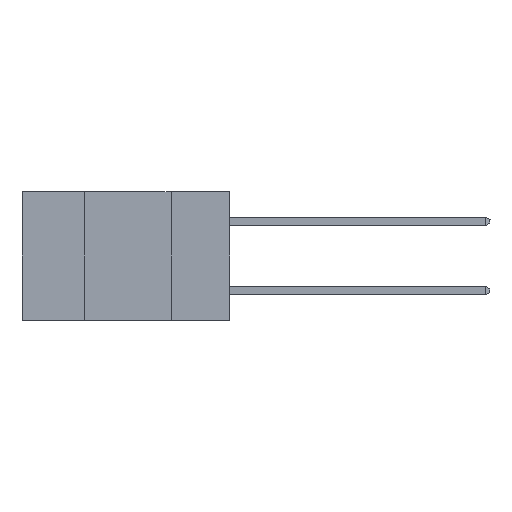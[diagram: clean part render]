
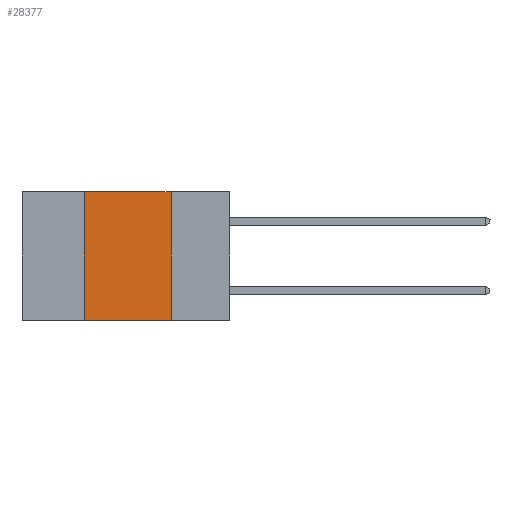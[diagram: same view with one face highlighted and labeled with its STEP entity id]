
A CAD part, left-side view. The second image highlights one B-rep face of the part: STEP entity #28377.
In plain terms, the highlighted planar face has unit normal (-1, 0, 0).
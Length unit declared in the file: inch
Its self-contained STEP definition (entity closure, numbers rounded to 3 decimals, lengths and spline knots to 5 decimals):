
#47 = PLANE ( 'NONE',  #2094 ) ;
#1327 = LINE ( 'NONE', #29027, #18824 ) ;
#1654 = CARTESIAN_POINT ( 'NONE',  ( 0., 0.17, -0.37 ) ) ;
#2094 = AXIS2_PLACEMENT_3D ( 'NONE', #13834, #7036, #9149 ) ;
#2950 = FACE_OUTER_BOUND ( 'NONE', #19973, .T. ) ;
#3147 = VERTEX_POINT ( 'NONE', #9108 ) ;
#4509 = ORIENTED_EDGE ( 'NONE', *, *, #16242, .F. ) ;
#6966 = VERTEX_POINT ( 'NONE', #1654 ) ;
#7036 = DIRECTION ( 'NONE',  ( 1., 0., 0. ) ) ;
#7650 = VECTOR ( 'NONE', #10135, 39.37008 ) ;
#9108 = CARTESIAN_POINT ( 'NONE',  ( 0., 0.42, -0.37 ) ) ;
#9149 = DIRECTION ( 'NONE',  ( 0., 0., -1. ) ) ;
#9240 = EDGE_CURVE ( 'NONE', #21513, #6966, #25194, .T. ) ;
#9243 = EDGE_CURVE ( 'NONE', #3147, #6966, #15176, .T. ) ;
#10068 = LINE ( 'NONE', #13271, #12910 ) ;
#10135 = DIRECTION ( 'NONE',  ( 0., -1., 0. ) ) ;
#12910 = VECTOR ( 'NONE', #22494, 39.37008 ) ;
#13271 = CARTESIAN_POINT ( 'NONE',  ( 0., 0.6, 0. ) ) ;
#13834 = CARTESIAN_POINT ( 'NONE',  ( 0., 0.6, 0. ) ) ;
#15176 = LINE ( 'NONE', #23714, #7650 ) ;
#15298 = DIRECTION ( 'NONE',  ( 0., 0., -1. ) ) ;
#16242 = EDGE_CURVE ( 'NONE', #22574, #21513, #10068, .T. ) ;
#18824 = VECTOR ( 'NONE', #28730, 39.37008 ) ;
#19582 = ORIENTED_EDGE ( 'NONE', *, *, #9240, .F. ) ;
#19973 = EDGE_LOOP ( 'NONE', ( #19582, #4509, #23894, #20174 ) ) ;
#20174 = ORIENTED_EDGE ( 'NONE', *, *, #9243, .T. ) ;
#20355 = EDGE_CURVE ( 'NONE', #3147, #22574, #1327, .T. ) ;
#21513 = VERTEX_POINT ( 'NONE', #26484 ) ;
#22494 = DIRECTION ( 'NONE',  ( 0., -1., 0. ) ) ;
#22574 = VERTEX_POINT ( 'NONE', #29484 ) ;
#23714 = CARTESIAN_POINT ( 'NONE',  ( 0., 0.6, -0.37 ) ) ;
#23894 = ORIENTED_EDGE ( 'NONE', *, *, #20355, .F. ) ;
#25194 = LINE ( 'NONE', #26677, #25877 ) ;
#25877 = VECTOR ( 'NONE', #15298, 39.37008 ) ;
#26484 = CARTESIAN_POINT ( 'NONE',  ( 0., 0.17, 0. ) ) ;
#26677 = CARTESIAN_POINT ( 'NONE',  ( 0., 0.17, 0. ) ) ;
#28377 = ADVANCED_FACE ( 'NONE', ( #2950 ), #47, .F. ) ;
#28730 = DIRECTION ( 'NONE',  ( 0., 0., 1. ) ) ;
#29027 = CARTESIAN_POINT ( 'NONE',  ( 0., 0.42, 0. ) ) ;
#29484 = CARTESIAN_POINT ( 'NONE',  ( 0., 0.42, 0. ) ) ;
